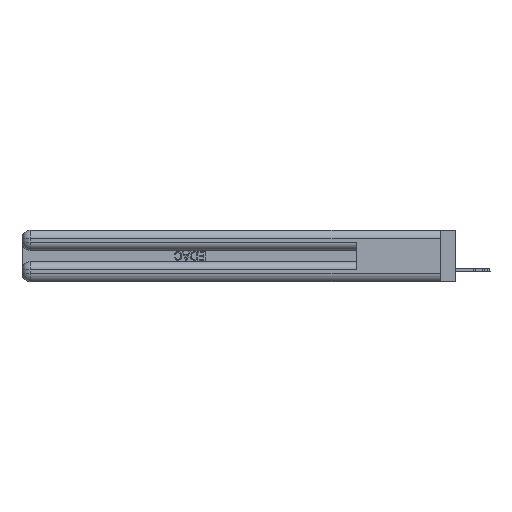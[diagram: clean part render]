
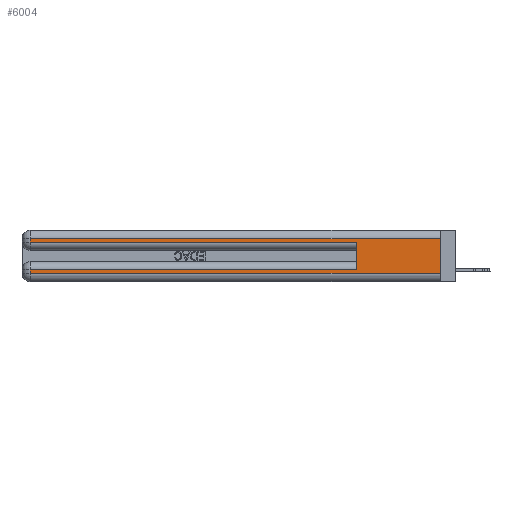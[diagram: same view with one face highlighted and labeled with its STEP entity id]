
A CAD part, left-side view. The second image highlights one B-rep face of the part: STEP entity #6004.
In plain terms, the highlighted planar face has unit normal (-1, 0, 0).
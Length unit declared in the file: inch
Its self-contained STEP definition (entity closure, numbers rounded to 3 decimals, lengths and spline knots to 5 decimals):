
#826 = CARTESIAN_POINT ( 'NONE',  ( 0., 0.6, 0.145 ) ) ;
#837 = CARTESIAN_POINT ( 'NONE',  ( 0., 2.94, 0.085 ) ) ;
#1416 = VERTEX_POINT ( 'NONE', #22909 ) ;
#2038 = VERTEX_POINT ( 'NONE', #15985 ) ;
#2753 = CARTESIAN_POINT ( 'NONE',  ( 0., 0., 0.37 ) ) ;
#5728 = CARTESIAN_POINT ( 'NONE',  ( 0., 2.94, 0.37 ) ) ;
#6004 = ADVANCED_FACE ( 'NONE', ( #38953 ), #49092, .F. ) ;
#6156 = VECTOR ( 'NONE', #35540, 39.37008 ) ;
#6376 = EDGE_CURVE ( 'NONE', #50719, #1416, #42336, .T. ) ;
#6728 = ORIENTED_EDGE ( 'NONE', *, *, #6915, .T. ) ;
#6915 = EDGE_CURVE ( 'NONE', #20179, #24403, #44872, .T. ) ;
#6982 = EDGE_CURVE ( 'NONE', #52740, #20179, #40173, .T. ) ;
#7489 = CARTESIAN_POINT ( 'NONE',  ( 0., 2.94, 0.31 ) ) ;
#7627 = VECTOR ( 'NONE', #15942, 39.37008 ) ;
#8853 = VECTOR ( 'NONE', #34756, 39.37008 ) ;
#8867 = CARTESIAN_POINT ( 'NONE',  ( 0., 2.94, 0.06 ) ) ;
#9321 = ORIENTED_EDGE ( 'NONE', *, *, #30791, .T. ) ;
#10472 = CARTESIAN_POINT ( 'NONE',  ( 0., 0.6, 0.285 ) ) ;
#10881 = EDGE_CURVE ( 'NONE', #35067, #30123, #18332, .T. ) ;
#11591 = DIRECTION ( 'NONE',  ( 0., 0., -1. ) ) ;
#15135 = LINE ( 'NONE', #30909, #53169 ) ;
#15942 = DIRECTION ( 'NONE',  ( 0., -1., 0. ) ) ;
#15985 = CARTESIAN_POINT ( 'NONE',  ( 0., 0.6, 0.085 ) ) ;
#16872 = DIRECTION ( 'NONE',  ( 0., 1., 0. ) ) ;
#18142 = VECTOR ( 'NONE', #19554, 39.37008 ) ;
#18332 = LINE ( 'NONE', #54549, #27773 ) ;
#19554 = DIRECTION ( 'NONE',  ( 0., 0., -1. ) ) ;
#20179 = VERTEX_POINT ( 'NONE', #28881 ) ;
#20720 = ORIENTED_EDGE ( 'NONE', *, *, #36430, .F. ) ;
#20956 = CARTESIAN_POINT ( 'NONE',  ( 0., 0., 0.31 ) ) ;
#22909 = CARTESIAN_POINT ( 'NONE',  ( 0., 0., 0.06 ) ) ;
#24403 = VERTEX_POINT ( 'NONE', #10472 ) ;
#24821 = ORIENTED_EDGE ( 'NONE', *, *, #6376, .F. ) ;
#26448 = CARTESIAN_POINT ( 'NONE',  ( 0., 0., 0.085 ) ) ;
#27727 = DIRECTION ( 'NONE',  ( 1., 0., 0. ) ) ;
#27773 = VECTOR ( 'NONE', #11591, 39.37008 ) ;
#28135 = LINE ( 'NONE', #826, #8853 ) ;
#28881 = CARTESIAN_POINT ( 'NONE',  ( 0., 2.94, 0.285 ) ) ;
#29486 = AXIS2_PLACEMENT_3D ( 'NONE', #53386, #27727, #48351 ) ;
#30123 = VERTEX_POINT ( 'NONE', #8867 ) ;
#30791 = EDGE_CURVE ( 'NONE', #30123, #1416, #15135, .T. ) ;
#30909 = CARTESIAN_POINT ( 'NONE',  ( 0., 0., 0.06 ) ) ;
#32678 = CARTESIAN_POINT ( 'NONE',  ( 0., 0., 0.285 ) ) ;
#33438 = LINE ( 'NONE', #26448, #43341 ) ;
#34164 = VECTOR ( 'NONE', #16872, 39.37008 ) ;
#34756 = DIRECTION ( 'NONE',  ( 0., 0., 1. ) ) ;
#34792 = LINE ( 'NONE', #20956, #34164 ) ;
#35067 = VERTEX_POINT ( 'NONE', #837 ) ;
#35262 = DIRECTION ( 'NONE',  ( 0., -1., 0. ) ) ;
#35540 = DIRECTION ( 'NONE',  ( 0., 0., -1. ) ) ;
#36430 = EDGE_CURVE ( 'NONE', #2038, #24403, #28135, .T. ) ;
#36923 = EDGE_CURVE ( 'NONE', #50719, #52740, #34792, .T. ) ;
#37603 = EDGE_CURVE ( 'NONE', #2038, #35067, #33438, .T. ) ;
#38953 = FACE_OUTER_BOUND ( 'NONE', #54281, .T. ) ;
#39231 = ORIENTED_EDGE ( 'NONE', *, *, #37603, .T. ) ;
#40173 = LINE ( 'NONE', #5728, #6156 ) ;
#42336 = LINE ( 'NONE', #2753, #18142 ) ;
#42470 = ORIENTED_EDGE ( 'NONE', *, *, #6982, .T. ) ;
#42700 = ORIENTED_EDGE ( 'NONE', *, *, #10881, .T. ) ;
#43319 = DIRECTION ( 'NONE',  ( 0., 1., 0. ) ) ;
#43341 = VECTOR ( 'NONE', #43319, 39.37008 ) ;
#43747 = CARTESIAN_POINT ( 'NONE',  ( 0., 0., 0.31 ) ) ;
#44128 = ORIENTED_EDGE ( 'NONE', *, *, #36923, .T. ) ;
#44872 = LINE ( 'NONE', #32678, #7627 ) ;
#48351 = DIRECTION ( 'NONE',  ( 0., 0., -1. ) ) ;
#49092 = PLANE ( 'NONE',  #29486 ) ;
#50719 = VERTEX_POINT ( 'NONE', #43747 ) ;
#52740 = VERTEX_POINT ( 'NONE', #7489 ) ;
#53169 = VECTOR ( 'NONE', #35262, 39.37008 ) ;
#53386 = CARTESIAN_POINT ( 'NONE',  ( 0., 0., 0.37 ) ) ;
#54281 = EDGE_LOOP ( 'NONE', ( #24821, #44128, #42470, #6728, #20720, #39231, #42700, #9321 ) ) ;
#54549 = CARTESIAN_POINT ( 'NONE',  ( 0., 2.94, 0.37 ) ) ;
